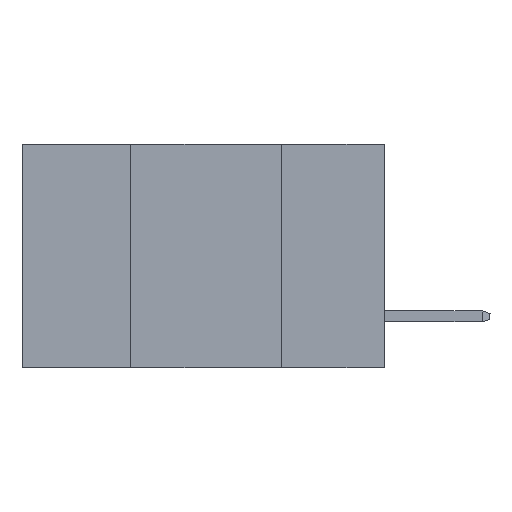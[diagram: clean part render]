
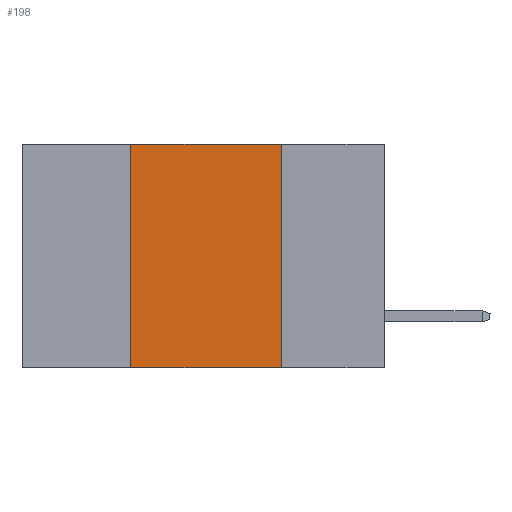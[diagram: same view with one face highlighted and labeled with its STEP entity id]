
A CAD part, left-side view. The second image highlights one B-rep face of the part: STEP entity #198.
In plain terms, the highlighted planar face has unit normal (-1, 0, 0).
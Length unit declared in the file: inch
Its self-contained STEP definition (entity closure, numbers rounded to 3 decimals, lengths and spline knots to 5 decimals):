
#165 = PLANE ( 'NONE',  #2012 ) ;
#198 = ADVANCED_FACE ( 'NONE', ( #281 ), #165, .F. ) ;
#281 = FACE_OUTER_BOUND ( 'NONE', #7779, .T. ) ;
#354 = VECTOR ( 'NONE', #8101, 39.37008 ) ;
#585 = VECTOR ( 'NONE', #2874, 39.37008 ) ;
#769 = LINE ( 'NONE', #8773, #3253 ) ;
#996 = EDGE_CURVE ( 'NONE', #1487, #10129, #8027, .T. ) ;
#1036 = CARTESIAN_POINT ( 'NONE',  ( 0., 0.42, -0.37 ) ) ;
#1263 = DIRECTION ( 'NONE',  ( 0., -1., 0. ) ) ;
#1487 = VERTEX_POINT ( 'NONE', #1036 ) ;
#2012 = AXIS2_PLACEMENT_3D ( 'NONE', #3840, #10930, #7361 ) ;
#2128 = CARTESIAN_POINT ( 'NONE',  ( 0., 0.17, 0. ) ) ;
#2707 = CARTESIAN_POINT ( 'NONE',  ( 0., 0.17, -0.37 ) ) ;
#2756 = CARTESIAN_POINT ( 'NONE',  ( 0., 0.42, -0.37 ) ) ;
#2874 = DIRECTION ( 'NONE',  ( 0., 0., 1. ) ) ;
#3253 = VECTOR ( 'NONE', #5301, 39.37008 ) ;
#3345 = EDGE_CURVE ( 'NONE', #10129, #7479, #9384, .T. ) ;
#3544 = ORIENTED_EDGE ( 'NONE', *, *, #10966, .F. ) ;
#3598 = LINE ( 'NONE', #3651, #354 ) ;
#3651 = CARTESIAN_POINT ( 'NONE',  ( 0., 0.6, -0.37 ) ) ;
#3840 = CARTESIAN_POINT ( 'NONE',  ( 0., 0.6, 0. ) ) ;
#5301 = DIRECTION ( 'NONE',  ( 0., 0., -1. ) ) ;
#5654 = ORIENTED_EDGE ( 'NONE', *, *, #996, .F. ) ;
#6475 = EDGE_CURVE ( 'NONE', #1487, #9410, #3598, .T. ) ;
#7361 = DIRECTION ( 'NONE',  ( 0., 0., -1. ) ) ;
#7479 = VERTEX_POINT ( 'NONE', #2128 ) ;
#7779 = EDGE_LOOP ( 'NONE', ( #3544, #8104, #5654, #8423 ) ) ;
#7923 = VECTOR ( 'NONE', #1263, 39.37008 ) ;
#8027 = LINE ( 'NONE', #2756, #585 ) ;
#8101 = DIRECTION ( 'NONE',  ( 0., -1., 0. ) ) ;
#8104 = ORIENTED_EDGE ( 'NONE', *, *, #3345, .F. ) ;
#8423 = ORIENTED_EDGE ( 'NONE', *, *, #6475, .T. ) ;
#8773 = CARTESIAN_POINT ( 'NONE',  ( 0., 0.17, -0.37 ) ) ;
#9384 = LINE ( 'NONE', #10074, #7923 ) ;
#9410 = VERTEX_POINT ( 'NONE', #2707 ) ;
#10074 = CARTESIAN_POINT ( 'NONE',  ( 0., 0.6, 0. ) ) ;
#10129 = VERTEX_POINT ( 'NONE', #10321 ) ;
#10321 = CARTESIAN_POINT ( 'NONE',  ( 0., 0.42, 0. ) ) ;
#10930 = DIRECTION ( 'NONE',  ( 1., 0., 0. ) ) ;
#10966 = EDGE_CURVE ( 'NONE', #7479, #9410, #769, .T. ) ;
